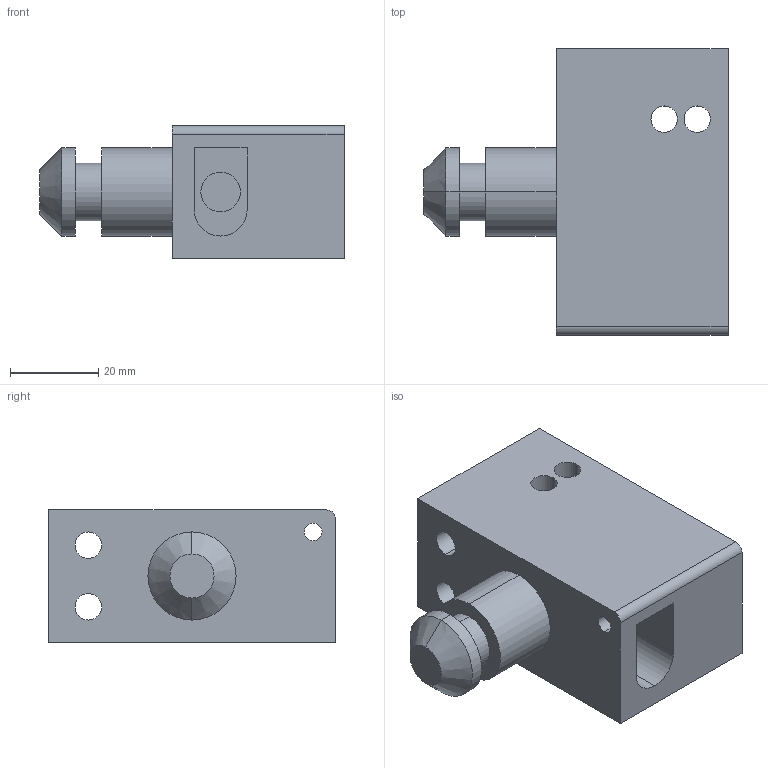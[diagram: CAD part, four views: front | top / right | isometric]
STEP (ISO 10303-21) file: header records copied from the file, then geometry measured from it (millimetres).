
FILE_DESCRIPTION (( 'STEP AP214' ), '1' );
FILE_NAME ('handle 2.0 5.56.STEP', '2025-05-18T10:37:44', ( '' ), ( '' ), 'SwSTEP 2.0', 'SolidWorks 2024', '' );
FILE_SCHEMA (( 'AUTOMOTIVE_DESIGN' ));
Length unit declared in the file: millimetre
Products named in the file (1): handle 2.0  5.56
Bounding box: 69 x 65 x 30 mm (x, y, z)
Volume: 69763.6 mm3; surface area: 18514.9 mm2
Topology: 1 solids, 1 shells, 38 faces, 97 edges, 64 vertices
Faces by surface type: cylinder 21, plane 15, cone 2
Entity records: 1220 total; most frequent: DIRECTION 223, CARTESIAN_POINT 200, ORIENTED_EDGE 194, EDGE_CURVE 97, AXIS2_PLACEMENT_3D 87, VERTEX_POINT 64, EDGE_LOOP 53, VECTOR 49
